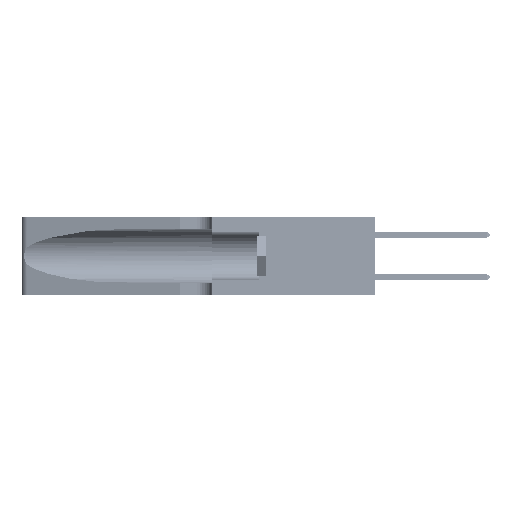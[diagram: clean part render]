
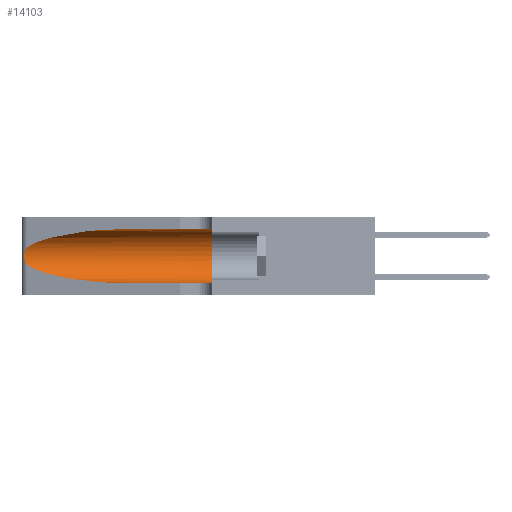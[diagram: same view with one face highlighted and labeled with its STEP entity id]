
A CAD part, left-side view. The second image highlights one B-rep face of the part: STEP entity #14103.
In plain terms, the highlighted cylindrical face has radius 3.308 mm (diameter 6.617 mm), a partial arc.
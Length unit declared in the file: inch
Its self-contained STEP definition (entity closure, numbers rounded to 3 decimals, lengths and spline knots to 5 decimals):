
#762 = ORIENTED_EDGE ( 'NONE', *, *, #46219, .F. ) ;
#1817 = EDGE_CURVE ( 'NONE', #6858, #8100, #27820, .T. ) ;
#3042 = CARTESIAN_POINT ( 'NONE',  ( 0.25854, 1.2359, 0.20912 ) ) ;
#3849 = CARTESIAN_POINT ( 'NONE',  ( 0.1305, 1.61858, 0.31525 ) ) ;
#4832 = B_SPLINE_CURVE_WITH_KNOTS ( 'NONE', 3,
 ( #48966, #24024, #53111, #28258, #3042, #32457, #7229, #36668, #11482, #40828, #15697, #44977, #19960, #49148 ),
 .UNSPECIFIED., .F., .F.,
 ( 4, 2, 2, 2, 2, 2, 4 ),
 ( 0., 0.00027, 0.00053, 0.00107, 0.0016, 0.00187, 0.00214 ),
 .UNSPECIFIED. ) ;
#5499 = LINE ( 'NONE', #8964, #26598 ) ;
#6354 = ORIENTED_EDGE ( 'NONE', *, *, #1817, .F. ) ;
#6858 = VERTEX_POINT ( 'NONE', #15006 ) ;
#7229 = CARTESIAN_POINT ( 'NONE',  ( 0.26075, 1.23896, 0.19203 ) ) ;
#8100 = VERTEX_POINT ( 'NONE', #23415 ) ;
#8496 = DIRECTION ( 'NONE',  ( 0., 1., 0. ) ) ;
#8608 = VERTEX_POINT ( 'NONE', #24738 ) ;
#8964 = CARTESIAN_POINT ( 'NONE',  ( 0.1305, 1.61858, 0.05475 ) ) ;
#11482 = CARTESIAN_POINT ( 'NONE',  ( 0.26017, 1.23833, 0.17102 ) ) ;
#11488 = VECTOR ( 'NONE', #37456, 39.37008 ) ;
#13069 = EDGE_CURVE ( 'NONE', #43532, #8608, #4832, .T. ) ;
#13601 = ORIENTED_EDGE ( 'NONE', *, *, #13069, .T. ) ;
#13663 =( BOUNDED_CURVE ( )  B_SPLINE_CURVE ( 3, ( #42268, #46415, #50566, #25659 ),
 .UNSPECIFIED., .F., .T. ) 
 B_SPLINE_CURVE_WITH_KNOTS ( ( 4, 4 ),
 ( 3.44316, 4.71239 ),
 .UNSPECIFIED. ) 
 CURVE ( )  GEOMETRIC_REPRESENTATION_ITEM ( )  RATIONAL_B_SPLINE_CURVE ( ( 1., 0.87, 0.87, 1. ) ) 
 REPRESENTATION_ITEM ( '' )  );
#13703 = VERTEX_POINT ( 'NONE', #48711 ) ;
#14103 = ADVANCED_FACE ( 'NONE', ( #25734 ), #35543, .F. ) ;
#15006 = CARTESIAN_POINT ( 'NONE',  ( 0.1305, 0.35, 0.31525 ) ) ;
#15697 = CARTESIAN_POINT ( 'NONE',  ( 0.25789, 1.23486, 0.15765 ) ) ;
#18783 = EDGE_CURVE ( 'NONE', #13703, #8100, #5499, .T. ) ;
#19960 = CARTESIAN_POINT ( 'NONE',  ( 0.25555, 1.22993, 0.14849 ) ) ;
#20801 = VERTEX_POINT ( 'NONE', #45527 ) ;
#23077 = CARTESIAN_POINT ( 'NONE',  ( 0.25487, 1.22718, 0.22369 ) ) ;
#23415 = CARTESIAN_POINT ( 'NONE',  ( 0.1305, 0.35, 0.05475 ) ) ;
#24024 = CARTESIAN_POINT ( 'NONE',  ( 0.25555, 1.22994, 0.2215 ) ) ;
#24738 = CARTESIAN_POINT ( 'NONE',  ( 0.25487, 1.22718, 0.14631 ) ) ;
#25659 = CARTESIAN_POINT ( 'NONE',  ( 0.1305, 0.72297, 0.05475 ) ) ;
#25734 = FACE_OUTER_BOUND ( 'NONE', #45031, .T. ) ;
#26472 = CARTESIAN_POINT ( 'NONE',  ( 0.1305, 1.61858, 0.185 ) ) ;
#26598 = VECTOR ( 'NONE', #42529, 39.37008 ) ;
#27057 = AXIS2_PLACEMENT_3D ( 'NONE', #33705, #8496, #37908 ) ;
#27300 = EDGE_CURVE ( 'NONE', #8608, #13703, #13663, .T. ) ;
#27820 = CIRCLE ( 'NONE', #27057, 0.13025 ) ;
#28258 = CARTESIAN_POINT ( 'NONE',  ( 0.25787, 1.23484, 0.2124 ) ) ;
#30700 = DIRECTION ( 'NONE',  ( 0., -1., 0. ) ) ;
#32061 = ORIENTED_EDGE ( 'NONE', *, *, #27300, .T. ) ;
#32261 = CARTESIAN_POINT ( 'NONE',  ( 0.25487, 1.22718, 0.22369 ) ) ;
#32457 = CARTESIAN_POINT ( 'NONE',  ( 0.26018, 1.23835, 0.19895 ) ) ;
#33705 = CARTESIAN_POINT ( 'NONE',  ( 0.1305, 0.35, 0.185 ) ) ;
#35543 = CYLINDRICAL_SURFACE ( 'NONE', #44312, 0.13025 ) ;
#36668 = CARTESIAN_POINT ( 'NONE',  ( 0.26075, 1.23896, 0.178 ) ) ;
#37456 = DIRECTION ( 'NONE',  ( 0., -1., 0. ) ) ;
#37908 = DIRECTION ( 'NONE',  ( 0., 0., 1. ) ) ;
#39730 = CARTESIAN_POINT ( 'NONE',  ( 0.18966, 0.96281, 0.31525 ) ) ;
#40456 =( BOUNDED_CURVE ( )  B_SPLINE_CURVE ( 3, ( #43889, #39730, #48024, #23077 ),
 .UNSPECIFIED., .F., .F. ) 
 B_SPLINE_CURVE_WITH_KNOTS ( ( 4, 4 ),
 ( 1.5708, 2.84003 ),
 .UNSPECIFIED. ) 
 CURVE ( )  GEOMETRIC_REPRESENTATION_ITEM ( )  RATIONAL_B_SPLINE_CURVE ( ( 1., 0.87, 0.87, 1. ) ) 
 REPRESENTATION_ITEM ( '' )  );
#40828 = CARTESIAN_POINT ( 'NONE',  ( 0.25856, 1.23593, 0.16098 ) ) ;
#42268 = CARTESIAN_POINT ( 'NONE',  ( 0.25487, 1.22718, 0.14631 ) ) ;
#42529 = DIRECTION ( 'NONE',  ( 0., -1., 0. ) ) ;
#43408 = EDGE_CURVE ( 'NONE', #20801, #43532, #40456, .T. ) ;
#43532 = VERTEX_POINT ( 'NONE', #32261 ) ;
#43586 = LINE ( 'NONE', #3849, #11488 ) ;
#43889 = CARTESIAN_POINT ( 'NONE',  ( 0.1305, 0.72297, 0.31525 ) ) ;
#44312 = AXIS2_PLACEMENT_3D ( 'NONE', #26472, #30700, #47201 ) ;
#44977 = CARTESIAN_POINT ( 'NONE',  ( 0.25639, 1.23186, 0.15144 ) ) ;
#45031 = EDGE_LOOP ( 'NONE', ( #54000, #13601, #32061, #46047, #6354, #762 ) ) ;
#45527 = CARTESIAN_POINT ( 'NONE',  ( 0.1305, 0.72297, 0.31525 ) ) ;
#46047 = ORIENTED_EDGE ( 'NONE', *, *, #18783, .T. ) ;
#46219 = EDGE_CURVE ( 'NONE', #20801, #6858, #43586, .T. ) ;
#46415 = CARTESIAN_POINT ( 'NONE',  ( 0.2373, 1.15595, 0.08982 ) ) ;
#47201 = DIRECTION ( 'NONE',  ( 0., 0., -1. ) ) ;
#48024 = CARTESIAN_POINT ( 'NONE',  ( 0.2373, 1.15595, 0.28018 ) ) ;
#48711 = CARTESIAN_POINT ( 'NONE',  ( 0.1305, 0.72297, 0.05475 ) ) ;
#48966 = CARTESIAN_POINT ( 'NONE',  ( 0.25487, 1.22718, 0.22369 ) ) ;
#49148 = CARTESIAN_POINT ( 'NONE',  ( 0.25487, 1.22718, 0.14631 ) ) ;
#50566 = CARTESIAN_POINT ( 'NONE',  ( 0.18966, 0.96281, 0.05475 ) ) ;
#53111 = CARTESIAN_POINT ( 'NONE',  ( 0.25639, 1.23184, 0.21858 ) ) ;
#54000 = ORIENTED_EDGE ( 'NONE', *, *, #43408, .T. ) ;
